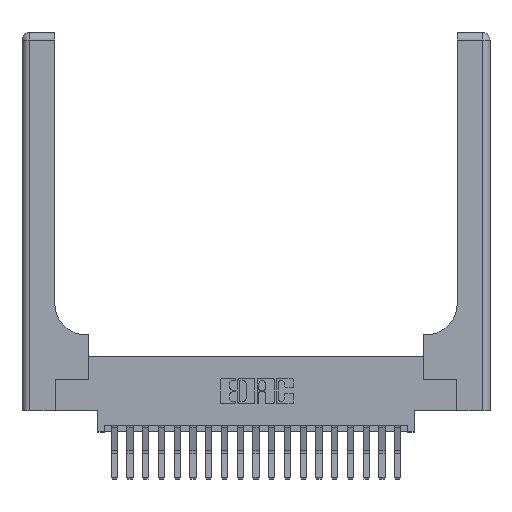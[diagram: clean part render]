
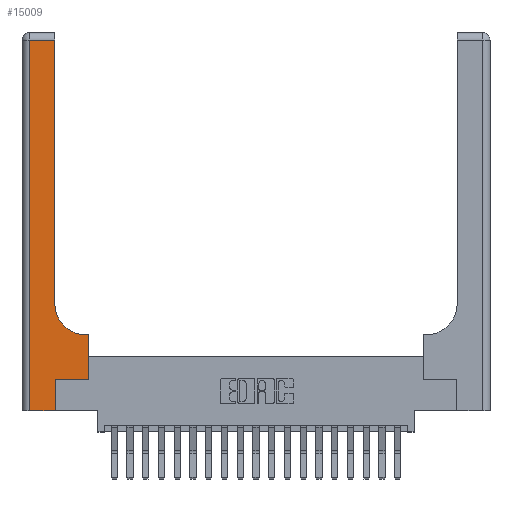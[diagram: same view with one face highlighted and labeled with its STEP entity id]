
A CAD part, top view. The second image highlights one B-rep face of the part: STEP entity #15009.
In plain terms, the highlighted planar face has unit normal (0, 0, 1).
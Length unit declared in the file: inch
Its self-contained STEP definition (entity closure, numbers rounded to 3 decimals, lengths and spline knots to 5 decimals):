
#139 = CARTESIAN_POINT ( 'NONE',  ( 0.26, 2.94, 0.37 ) ) ;
#567 = VERTEX_POINT ( 'NONE', #4827 ) ;
#804 = ORIENTED_EDGE ( 'NONE', *, *, #1915, .T. ) ;
#884 = LINE ( 'NONE', #7681, #6839 ) ;
#917 = LINE ( 'NONE', #2320, #15837 ) ;
#1011 = CARTESIAN_POINT ( 'NONE',  ( 0.528, 0.25, 0.37 ) ) ;
#1423 = CARTESIAN_POINT ( 'NONE',  ( 0.51, 0.85, 0.37 ) ) ;
#1534 = DIRECTION ( 'NONE',  ( 0., 0., -1. ) ) ;
#1915 = EDGE_CURVE ( 'NONE', #8114, #4586, #917, .T. ) ;
#1928 = VECTOR ( 'NONE', #13455, 39.37008 ) ;
#2156 = CARTESIAN_POINT ( 'NONE',  ( 0., 3., 0.37 ) ) ;
#2271 = ORIENTED_EDGE ( 'NONE', *, *, #13398, .T. ) ;
#2320 = CARTESIAN_POINT ( 'NONE',  ( 0.26, 3., 0.37 ) ) ;
#2522 = DIRECTION ( 'NONE',  ( 0., 1., 0. ) ) ;
#2611 = DIRECTION ( 'NONE',  ( 0., 1., 0. ) ) ;
#2685 = VECTOR ( 'NONE', #2522, 39.37008 ) ;
#2862 = LINE ( 'NONE', #14400, #18041 ) ;
#3036 = DIRECTION ( 'NONE',  ( 1., 0., 0. ) ) ;
#3281 = DIRECTION ( 'NONE',  ( 1., 0., 0. ) ) ;
#3674 = VERTEX_POINT ( 'NONE', #7807 ) ;
#4586 = VERTEX_POINT ( 'NONE', #139 ) ;
#4827 = CARTESIAN_POINT ( 'NONE',  ( 0.265, 0.25, 0.37 ) ) ;
#5291 = EDGE_CURVE ( 'NONE', #19078, #14017, #2862, .T. ) ;
#5369 = LINE ( 'NONE', #6885, #1928 ) ;
#5672 = DIRECTION ( 'NONE',  ( 1., 0., 0. ) ) ;
#5761 = EDGE_LOOP ( 'NONE', ( #804, #20275, #12265, #6712, #2271, #16092, #7619, #9266, #20157 ) ) ;
#5981 = LINE ( 'NONE', #1011, #2685 ) ;
#6009 = DIRECTION ( 'NONE',  ( -1., 0., 0. ) ) ;
#6712 = ORIENTED_EDGE ( 'NONE', *, *, #5291, .T. ) ;
#6821 = PLANE ( 'NONE',  #13762 ) ;
#6839 = VECTOR ( 'NONE', #2611, 39.37008 ) ;
#6885 = CARTESIAN_POINT ( 'NONE',  ( 0.26, 0.6, 0.37 ) ) ;
#6920 = CARTESIAN_POINT ( 'NONE',  ( 0.528, 0.25, 0.37 ) ) ;
#7117 = DIRECTION ( 'NONE',  ( 0., -1., 0. ) ) ;
#7170 = CARTESIAN_POINT ( 'NONE',  ( 0.06, 2.94, 0.37 ) ) ;
#7227 = DIRECTION ( 'NONE',  ( 0., 0., -1. ) ) ;
#7619 = ORIENTED_EDGE ( 'NONE', *, *, #12988, .T. ) ;
#7681 = CARTESIAN_POINT ( 'NONE',  ( 0.265, 0., 0.37 ) ) ;
#7807 = CARTESIAN_POINT ( 'NONE',  ( 0.51, 0.6, 0.37 ) ) ;
#7842 = VERTEX_POINT ( 'NONE', #20931 ) ;
#8114 = VERTEX_POINT ( 'NONE', #20650 ) ;
#8194 = VECTOR ( 'NONE', #6009, 39.37008 ) ;
#9266 = ORIENTED_EDGE ( 'NONE', *, *, #10530, .T. ) ;
#9714 = VECTOR ( 'NONE', #7117, 39.37008 ) ;
#10239 = CARTESIAN_POINT ( 'NONE',  ( 0.06, 3., 0.37 ) ) ;
#10530 = EDGE_CURVE ( 'NONE', #7842, #3674, #5369, .T. ) ;
#10846 = DIRECTION ( 'NONE',  ( 0., 1., 0. ) ) ;
#11126 = EDGE_CURVE ( 'NONE', #567, #15003, #14709, .T. ) ;
#11287 = CARTESIAN_POINT ( 'NONE',  ( 0.265, 0., 0.37 ) ) ;
#11357 = CARTESIAN_POINT ( 'NONE',  ( 0.265, 0.25, 0.37 ) ) ;
#11872 = FACE_OUTER_BOUND ( 'NONE', #5761, .T. ) ;
#12265 = ORIENTED_EDGE ( 'NONE', *, *, #20277, .T. ) ;
#12346 = AXIS2_PLACEMENT_3D ( 'NONE', #1423, #1534, #3036 ) ;
#12480 = CARTESIAN_POINT ( 'NONE',  ( 0., 2.94, 0.37 ) ) ;
#12606 = EDGE_CURVE ( 'NONE', #4586, #12748, #14092, .T. ) ;
#12748 = VERTEX_POINT ( 'NONE', #7170 ) ;
#12988 = EDGE_CURVE ( 'NONE', #15003, #7842, #5981, .T. ) ;
#13398 = EDGE_CURVE ( 'NONE', #14017, #567, #884, .T. ) ;
#13455 = DIRECTION ( 'NONE',  ( -1., 0., 0. ) ) ;
#13490 = DIRECTION ( 'NONE',  ( -1., 0., 0. ) ) ;
#13520 = EDGE_CURVE ( 'NONE', #3674, #8114, #14073, .T. ) ;
#13762 = AXIS2_PLACEMENT_3D ( 'NONE', #2156, #7227, #13490 ) ;
#14017 = VERTEX_POINT ( 'NONE', #11287 ) ;
#14073 = CIRCLE ( 'NONE', #12346, 0.25 ) ;
#14092 = LINE ( 'NONE', #12480, #8194 ) ;
#14400 = CARTESIAN_POINT ( 'NONE',  ( 0., 0., 0.37 ) ) ;
#14709 = LINE ( 'NONE', #11357, #17099 ) ;
#15003 = VERTEX_POINT ( 'NONE', #6920 ) ;
#15009 = ADVANCED_FACE ( 'NONE', ( #11872 ), #6821, .F. ) ;
#15837 = VECTOR ( 'NONE', #10846, 39.37008 ) ;
#16092 = ORIENTED_EDGE ( 'NONE', *, *, #11126, .T. ) ;
#17099 = VECTOR ( 'NONE', #3281, 39.37008 ) ;
#17441 = CARTESIAN_POINT ( 'NONE',  ( 0.06, 0., 0.37 ) ) ;
#18041 = VECTOR ( 'NONE', #5672, 39.37008 ) ;
#19078 = VERTEX_POINT ( 'NONE', #17441 ) ;
#20157 = ORIENTED_EDGE ( 'NONE', *, *, #13520, .T. ) ;
#20275 = ORIENTED_EDGE ( 'NONE', *, *, #12606, .T. ) ;
#20277 = EDGE_CURVE ( 'NONE', #12748, #19078, #20394, .T. ) ;
#20394 = LINE ( 'NONE', #10239, #9714 ) ;
#20650 = CARTESIAN_POINT ( 'NONE',  ( 0.26, 0.85, 0.37 ) ) ;
#20931 = CARTESIAN_POINT ( 'NONE',  ( 0.528, 0.6, 0.37 ) ) ;
